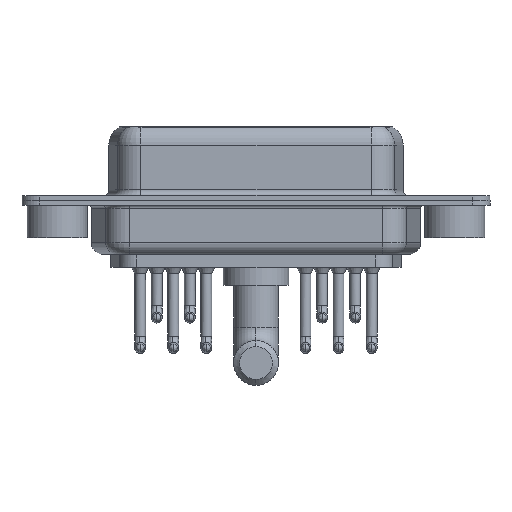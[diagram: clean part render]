
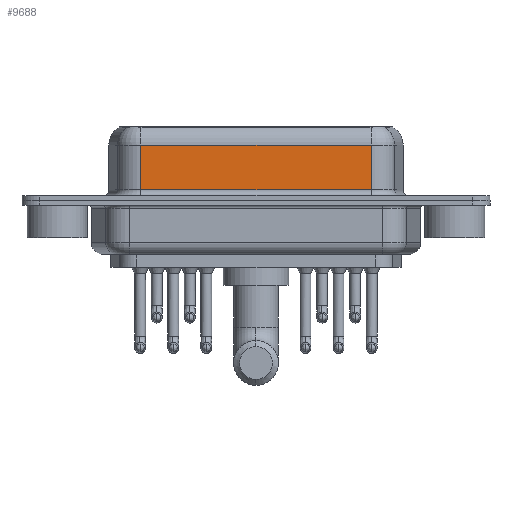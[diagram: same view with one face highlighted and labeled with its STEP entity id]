
A CAD part, front view. The second image highlights one B-rep face of the part: STEP entity #9688.
In plain terms, the highlighted planar face has unit normal (0, -1, 0).
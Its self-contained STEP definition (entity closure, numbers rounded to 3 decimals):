
#435 = ORIENTED_EDGE ( 'NONE', *, *, #16369, .T. ) ;
#460 = LINE ( 'NONE', #17909, #14938 ) ;
#1163 = CARTESIAN_POINT ( 'NONE',  ( 26.287, -3.95, 4.65 ) ) ;
#1253 = VERTEX_POINT ( 'NONE', #1163 ) ;
#2194 = VERTEX_POINT ( 'NONE', #14273 ) ;
#2785 = CARTESIAN_POINT ( 'NONE',  ( 26.287, -3.95, 6.4 ) ) ;
#2863 = ORIENTED_EDGE ( 'NONE', *, *, #2944, .T. ) ;
#2944 = EDGE_CURVE ( 'NONE', #8199, #2194, #9053, .T. ) ;
#3180 = VERTEX_POINT ( 'NONE', #5437 ) ;
#3807 = FACE_OUTER_BOUND ( 'NONE', #10031, .T. ) ;
#5437 = CARTESIAN_POINT ( 'NONE',  ( 26.287, -3.95, 0.9 ) ) ;
#5808 = EDGE_CURVE ( 'NONE', #1253, #3180, #8475, .T. ) ;
#6200 = DIRECTION ( 'NONE',  ( 0., 0., -1. ) ) ;
#6969 = DIRECTION ( 'NONE',  ( 0., 0., -1. ) ) ;
#7503 = DIRECTION ( 'NONE',  ( -1., 0., 0. ) ) ;
#8149 = ORIENTED_EDGE ( 'NONE', *, *, #14121, .T. ) ;
#8199 = VERTEX_POINT ( 'NONE', #9379 ) ;
#8356 = PLANE ( 'NONE',  #16902 ) ;
#8475 = LINE ( 'NONE', #2785, #16466 ) ;
#8960 = VECTOR ( 'NONE', #6200, 1000. ) ;
#9053 = LINE ( 'NONE', #13475, #8960 ) ;
#9379 = CARTESIAN_POINT ( 'NONE',  ( 7.013, -3.95, 4.65 ) ) ;
#9590 = CARTESIAN_POINT ( 'NONE',  ( 26.287, -3.95, 6.4 ) ) ;
#9688 = ADVANCED_FACE ( 'NONE', ( #3807 ), #8356, .F. ) ;
#10031 = EDGE_LOOP ( 'NONE', ( #11277, #8149, #2863, #435 ) ) ;
#10241 = CARTESIAN_POINT ( 'NONE',  ( 26.287, -3.95, 4.65 ) ) ;
#11277 = ORIENTED_EDGE ( 'NONE', *, *, #5808, .F. ) ;
#13383 = VECTOR ( 'NONE', #7503, 1000. ) ;
#13475 = CARTESIAN_POINT ( 'NONE',  ( 7.013, -3.95, 6.4 ) ) ;
#14121 = EDGE_CURVE ( 'NONE', #1253, #8199, #15966, .T. ) ;
#14273 = CARTESIAN_POINT ( 'NONE',  ( 7.013, -3.95, 0.9 ) ) ;
#14938 = VECTOR ( 'NONE', #16307, 1000. ) ;
#15697 = DIRECTION ( 'NONE',  ( 0., 1., 0. ) ) ;
#15966 = LINE ( 'NONE', #10241, #13383 ) ;
#16307 = DIRECTION ( 'NONE',  ( 1., 0., 0. ) ) ;
#16369 = EDGE_CURVE ( 'NONE', #2194, #3180, #460, .T. ) ;
#16466 = VECTOR ( 'NONE', #6969, 1000. ) ;
#16902 = AXIS2_PLACEMENT_3D ( 'NONE', #9590, #15697, #18241 ) ;
#17909 = CARTESIAN_POINT ( 'NONE',  ( 26.287, -3.95, 0.9 ) ) ;
#18241 = DIRECTION ( 'NONE',  ( 0., 0., 1. ) ) ;
